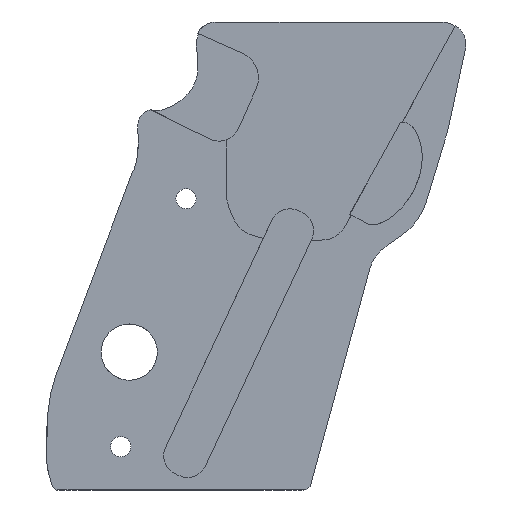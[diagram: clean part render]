
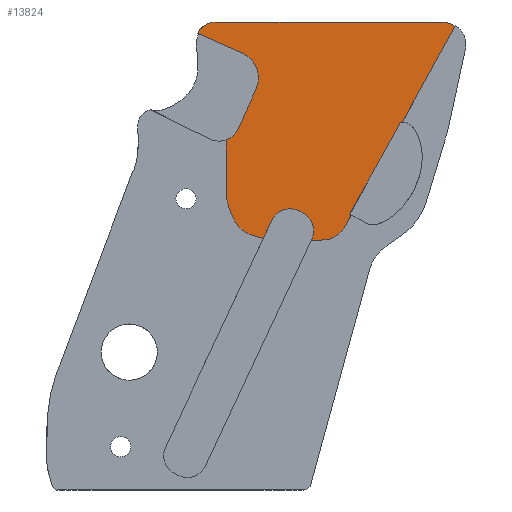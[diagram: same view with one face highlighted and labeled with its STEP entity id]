
A CAD part, front view. The second image highlights one B-rep face of the part: STEP entity #13824.
In plain terms, the highlighted planar face has unit normal (0, -1, 0).
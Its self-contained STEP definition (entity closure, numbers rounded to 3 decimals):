
#549=CIRCLE('',#14365,3.233);
#551=CIRCLE('',#14369,4.024);
#557=CIRCLE('',#14378,3.);
#558=CIRCLE('',#14379,3.);
#1231=B_SPLINE_CURVE_WITH_KNOTS('',3,(#36720,#36721,#36722,#36723,#36724),
 .UNSPECIFIED.,.F.,.F.,(4,1,4),(-0.348,-0.199,0.),
 .UNSPECIFIED.);
#1232=B_SPLINE_CURVE_WITH_KNOTS('',5,(#36728,#36729,#36730,#36731,#36732,
#36733,#36734,#36735,#36736,#36737,#36738,#36739,#36740,#36741,#36742),
 .UNSPECIFIED.,.F.,.F.,(6,1,1,1,1,1,1,1,1,1,6),(-1.,-0.9,-0.8,-0.7,-0.6,
-0.5,-0.4,-0.3,-0.2,-0.1,0.),.UNSPECIFIED.);
#1233=B_SPLINE_CURVE_WITH_KNOTS('',5,(#36754,#36755,#36756,#36757,#36758,
#36759,#36760,#36761,#36762,#36763,#36764,#36765,#36766,#36767,#36768),
 .UNSPECIFIED.,.F.,.F.,(6,1,1,1,1,1,1,1,1,1,6),(-1.,-0.9,-0.8,-0.7,-0.6,
-0.5,-0.4,-0.3,-0.2,-0.1,0.),.UNSPECIFIED.);
#1234=B_SPLINE_CURVE_WITH_KNOTS('',3,(#36772,#36773,#36774,#36775,#36776,
#36777),.UNSPECIFIED.,.F.,.F.,(4,2,4),(0.,0.115,0.23),
 .UNSPECIFIED.);
#1961=FACE_OUTER_BOUND('',#2740,.T.);
#2740=EDGE_LOOP('',(#12610,#12611,#12612,#12613,#12614,#12615,#12616,#12617,
#12618,#12619,#12620,#12621,#12622,#12623,#12624,#12625));
#3965=LINE('',#36233,#5205);
#3968=LINE('',#36241,#5208);
#3979=LINE('',#36726,#5219);
#3980=LINE('',#36744,#5220);
#3981=LINE('',#36748,#5221);
#3982=LINE('',#36752,#5222);
#3983=LINE('',#36770,#5223);
#3984=LINE('',#36778,#5224);
#5205=VECTOR('',#16616,10.);
#5208=VECTOR('',#16625,10.);
#5219=VECTOR('',#16650,10.);
#5220=VECTOR('',#16651,10.);
#5221=VECTOR('',#16654,10.);
#5222=VECTOR('',#16657,10.);
#5223=VECTOR('',#16658,10.);
#5224=VECTOR('',#16659,10.);
#6537=VERTEX_POINT('',#36225);
#6538=VERTEX_POINT('',#36227);
#6539=VERTEX_POINT('',#36232);
#6540=VERTEX_POINT('',#36236);
#6541=VERTEX_POINT('',#36240);
#6559=VERTEX_POINT('',#36719);
#6560=VERTEX_POINT('',#36725);
#6561=VERTEX_POINT('',#36727);
#6562=VERTEX_POINT('',#36743);
#6563=VERTEX_POINT('',#36745);
#6564=VERTEX_POINT('',#36747);
#6565=VERTEX_POINT('',#36749);
#6566=VERTEX_POINT('',#36751);
#6567=VERTEX_POINT('',#36753);
#6568=VERTEX_POINT('',#36769);
#6569=VERTEX_POINT('',#36771);
#8555=EDGE_CURVE('',#6537,#6538,#549,.T.);
#8558=EDGE_CURVE('',#6538,#6539,#3965,.T.);
#8560=EDGE_CURVE('',#6539,#6540,#551,.T.);
#8562=EDGE_CURVE('',#6540,#6541,#3968,.T.);
#8590=EDGE_CURVE('',#6541,#6559,#1231,.T.);
#8591=EDGE_CURVE('',#6560,#6537,#3979,.T.);
#8592=EDGE_CURVE('',#6561,#6560,#1232,.T.);
#8593=EDGE_CURVE('',#6562,#6561,#3980,.T.);
#8594=EDGE_CURVE('',#6563,#6562,#557,.T.);
#8595=EDGE_CURVE('',#6564,#6563,#3981,.T.);
#8596=EDGE_CURVE('',#6565,#6564,#558,.T.);
#8597=EDGE_CURVE('',#6566,#6565,#3982,.T.);
#8598=EDGE_CURVE('',#6567,#6566,#1233,.T.);
#8599=EDGE_CURVE('',#6568,#6567,#3983,.T.);
#8600=EDGE_CURVE('',#6569,#6568,#1234,.T.);
#8601=EDGE_CURVE('',#6559,#6569,#3984,.T.);
#12610=ORIENTED_EDGE('',*,*,#8590,.F.);
#12611=ORIENTED_EDGE('',*,*,#8562,.F.);
#12612=ORIENTED_EDGE('',*,*,#8560,.F.);
#12613=ORIENTED_EDGE('',*,*,#8558,.F.);
#12614=ORIENTED_EDGE('',*,*,#8555,.F.);
#12615=ORIENTED_EDGE('',*,*,#8591,.F.);
#12616=ORIENTED_EDGE('',*,*,#8592,.F.);
#12617=ORIENTED_EDGE('',*,*,#8593,.F.);
#12618=ORIENTED_EDGE('',*,*,#8594,.F.);
#12619=ORIENTED_EDGE('',*,*,#8595,.F.);
#12620=ORIENTED_EDGE('',*,*,#8596,.F.);
#12621=ORIENTED_EDGE('',*,*,#8597,.F.);
#12622=ORIENTED_EDGE('',*,*,#8598,.F.);
#12623=ORIENTED_EDGE('',*,*,#8599,.F.);
#12624=ORIENTED_EDGE('',*,*,#8600,.F.);
#12625=ORIENTED_EDGE('',*,*,#8601,.F.);
#13091=PLANE('',#14377);
#13824=ADVANCED_FACE('',(#1961),#13091,.F.);
#14365=AXIS2_PLACEMENT_3D('',#36228,#16609,#16610);
#14369=AXIS2_PLACEMENT_3D('',#36237,#16620,#16621);
#14377=AXIS2_PLACEMENT_3D('',#36718,#16648,#16649);
#14378=AXIS2_PLACEMENT_3D('',#36746,#16652,#16653);
#14379=AXIS2_PLACEMENT_3D('',#36750,#16655,#16656);
#16609=DIRECTION('center_axis',(0.,-1.,0.));
#16610=DIRECTION('ref_axis',(0.913,0.,-0.408));
#16616=DIRECTION('',(0.408,0.,0.913));
#16620=DIRECTION('center_axis',(0.,-1.,0.));
#16621=DIRECTION('ref_axis',(0.41,0.,0.912));
#16625=DIRECTION('',(-0.912,0.,0.41));
#16648=DIRECTION('center_axis',(0.,1.,0.));
#16649=DIRECTION('ref_axis',(1.,0.,0.));
#16650=DIRECTION('',(0.,0.,1.));
#16651=DIRECTION('',(-0.424,0.,-0.906));
#16652=DIRECTION('center_axis',(0.,-1.,0.));
#16653=DIRECTION('ref_axis',(-0.906,0.,0.424));
#16654=DIRECTION('',(-0.906,0.,0.424));
#16655=DIRECTION('center_axis',(0.,-1.,0.));
#16656=DIRECTION('ref_axis',(0.424,0.,0.906));
#16657=DIRECTION('',(0.424,0.,0.906));
#16658=DIRECTION('',(-0.482,0.,-0.876));
#16659=DIRECTION('',(1.,0.,0.));
#36225=CARTESIAN_POINT('',(8.558,0.55,14.984));
#36227=CARTESIAN_POINT('',(10.423,0.55,16.71));
#36228=CARTESIAN_POINT('Origin',(7.472,0.55,18.029));
#36232=CARTESIAN_POINT('',(13.056,0.55,22.6));
#36233=CARTESIAN_POINT('',(10.423,0.55,16.71));
#36236=CARTESIAN_POINT('',(11.032,0.55,27.912));
#36237=CARTESIAN_POINT('Origin',(9.382,0.55,24.242));
#36240=CARTESIAN_POINT('',(4.309,0.55,30.935));
#36241=CARTESIAN_POINT('',(11.032,0.55,27.912));
#36718=CARTESIAN_POINT('Origin',(22.703,0.55,16.907));
#36719=CARTESIAN_POINT('',(7.172,0.55,32.594));
#36720=CARTESIAN_POINT('Ctrl Pts',(4.309,0.55,30.935));
#36721=CARTESIAN_POINT('Ctrl Pts',(4.555,0.55,31.365));
#36722=CARTESIAN_POINT('Ctrl Pts',(5.359,0.55,32.237));
#36723=CARTESIAN_POINT('Ctrl Pts',(6.512,0.55,32.594));
#36724=CARTESIAN_POINT('Ctrl Pts',(7.172,0.55,32.594));
#36725=CARTESIAN_POINT('',(8.558,0.55,6.483));
#36726=CARTESIAN_POINT('',(8.558,0.55,14.984));
#36727=CARTESIAN_POINT('',(14.115,0.55,0.238));
#36728=CARTESIAN_POINT('Ctrl Pts',(14.115,0.55,0.238));
#36729=CARTESIAN_POINT('Ctrl Pts',(13.94,0.55,0.284));
#36730=CARTESIAN_POINT('Ctrl Pts',(13.597,0.55,0.375));
#36731=CARTESIAN_POINT('Ctrl Pts',(13.104,0.55,0.51));
#36732=CARTESIAN_POINT('Ctrl Pts',(12.49,0.55,0.694));
#36733=CARTESIAN_POINT('Ctrl Pts',(11.793,0.55,0.966));
#36734=CARTESIAN_POINT('Ctrl Pts',(11.164,0.55,1.323));
#36735=CARTESIAN_POINT('Ctrl Pts',(10.599,0.55,1.807));
#36736=CARTESIAN_POINT('Ctrl Pts',(10.094,0.55,2.443));
#36737=CARTESIAN_POINT('Ctrl Pts',(9.642,0.55,3.232));
#36738=CARTESIAN_POINT('Ctrl Pts',(9.237,0.55,4.169));
#36739=CARTESIAN_POINT('Ctrl Pts',(8.946,0.55,5.03));
#36740=CARTESIAN_POINT('Ctrl Pts',(8.745,0.55,5.734));
#36741=CARTESIAN_POINT('Ctrl Pts',(8.619,0.55,6.229));
#36742=CARTESIAN_POINT('Ctrl Pts',(8.558,0.55,6.483));
#36743=CARTESIAN_POINT('',(15.383,0.55,2.946));
#36744=CARTESIAN_POINT('',(10.793,0.55,-6.857));
#36745=CARTESIAN_POINT('',(19.372,0.55,4.39));
#36746=CARTESIAN_POINT('Origin',(18.1,0.55,1.673));
#36747=CARTESIAN_POINT('',(19.924,0.55,4.132));
#36748=CARTESIAN_POINT('',(18.334,0.55,4.876));
#36749=CARTESIAN_POINT('',(21.369,0.55,0.143));
#36750=CARTESIAN_POINT('Origin',(18.652,0.55,1.415));
#36751=CARTESIAN_POINT('',(21.286,0.55,-0.035));
#36752=CARTESIAN_POINT('',(24.708,0.55,7.273));
#36753=CARTESIAN_POINT('',(26.317,0.55,2.057));
#36754=CARTESIAN_POINT('Ctrl Pts',(26.317,0.55,2.057));
#36755=CARTESIAN_POINT('Ctrl Pts',(26.283,0.55,1.99));
#36756=CARTESIAN_POINT('Ctrl Pts',(26.203,0.55,1.85));
#36757=CARTESIAN_POINT('Ctrl Pts',(26.045,0.55,1.62));
#36758=CARTESIAN_POINT('Ctrl Pts',(25.763,0.55,1.286));
#36759=CARTESIAN_POINT('Ctrl Pts',(25.319,0.55,0.866));
#36760=CARTESIAN_POINT('Ctrl Pts',(24.818,0.55,0.497));
#36761=CARTESIAN_POINT('Ctrl Pts',(24.289,0.55,0.226));
#36762=CARTESIAN_POINT('Ctrl Pts',(23.749,0.55,0.073));
#36763=CARTESIAN_POINT('Ctrl Pts',(23.196,0.55,0.017));
#36764=CARTESIAN_POINT('Ctrl Pts',(22.615,0.55,0.013));
#36765=CARTESIAN_POINT('Ctrl Pts',(22.115,0.55,0.014));
#36766=CARTESIAN_POINT('Ctrl Pts',(21.712,0.55,-0.002));
#36767=CARTESIAN_POINT('Ctrl Pts',(21.43,0.55,-0.023));
#36768=CARTESIAN_POINT('Ctrl Pts',(21.286,0.55,-0.035));
#36769=CARTESIAN_POINT('',(42.784,0.55,31.965));
#36770=CARTESIAN_POINT('',(26.317,0.55,2.057));
#36771=CARTESIAN_POINT('',(40.621,0.55,32.594));
#36772=CARTESIAN_POINT('Ctrl Pts',(40.621,0.55,32.594));
#36773=CARTESIAN_POINT('Ctrl Pts',(41.004,0.55,32.594));
#36774=CARTESIAN_POINT('Ctrl Pts',(41.384,0.55,32.545));
#36775=CARTESIAN_POINT('Ctrl Pts',(42.119,0.55,32.337));
#36776=CARTESIAN_POINT('Ctrl Pts',(42.466,0.55,32.179));
#36777=CARTESIAN_POINT('Ctrl Pts',(42.784,0.55,31.965));
#36778=CARTESIAN_POINT('',(8.985,0.55,32.594));
